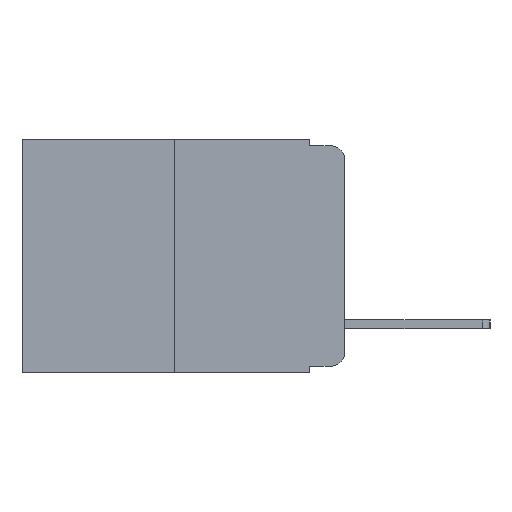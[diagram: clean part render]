
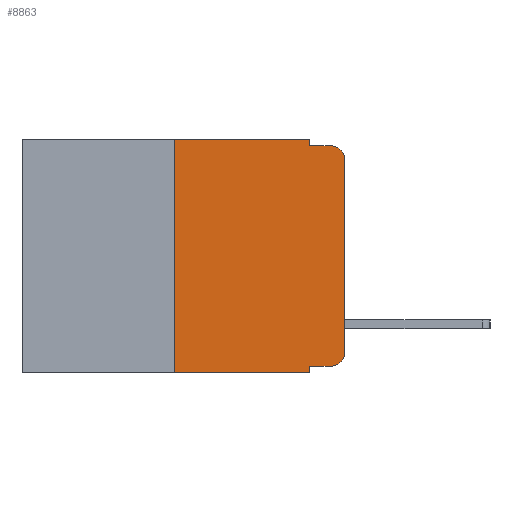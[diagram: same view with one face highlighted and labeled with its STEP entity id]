
A CAD part, left-side view. The second image highlights one B-rep face of the part: STEP entity #8863.
In plain terms, the highlighted planar face has unit normal (-1, 0, 0).
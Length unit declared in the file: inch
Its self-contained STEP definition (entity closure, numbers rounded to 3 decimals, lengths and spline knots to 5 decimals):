
#88 = EDGE_CURVE ( 'NONE', #5601, #2512, #3696, .T. ) ;
#154 = CARTESIAN_POINT ( 'NONE',  ( 0., 0., -0.313 ) ) ;
#872 = CARTESIAN_POINT ( 'NONE',  ( 0., 0.051, -0.343 ) ) ;
#1661 = EDGE_CURVE ( 'NONE', #13892, #5601, #1876, .T. ) ;
#1876 = LINE ( 'NONE', #6268, #14710 ) ;
#1945 = DIRECTION ( 'NONE',  ( 1., 0., 0. ) ) ;
#2285 = VERTEX_POINT ( 'NONE', #15141 ) ;
#2512 = VERTEX_POINT ( 'NONE', #3735 ) ;
#2529 = VECTOR ( 'NONE', #13108, 39.37008 ) ;
#2612 = AXIS2_PLACEMENT_3D ( 'NONE', #18096, #9336, #19507 ) ;
#2940 = CARTESIAN_POINT ( 'NONE',  ( 0., 0.051, 0. ) ) ;
#3211 = VECTOR ( 'NONE', #10409, 39.37008 ) ;
#3261 = AXIS2_PLACEMENT_3D ( 'NONE', #14001, #4772, #15434 ) ;
#3561 = ORIENTED_EDGE ( 'NONE', *, *, #1661, .F. ) ;
#3588 = CARTESIAN_POINT ( 'NONE',  ( 0., 0.473, -0.343 ) ) ;
#3696 = LINE ( 'NONE', #9716, #3211 ) ;
#3728 = CARTESIAN_POINT ( 'NONE',  ( 0., 0.051, 0. ) ) ;
#3735 = CARTESIAN_POINT ( 'NONE',  ( 0., 0.051, -0.01 ) ) ;
#3937 = CARTESIAN_POINT ( 'NONE',  ( 0., 0.02, -0.01 ) ) ;
#4514 = VERTEX_POINT ( 'NONE', #154 ) ;
#4584 = DIRECTION ( 'NONE',  ( 0., 0., 1. ) ) ;
#4772 = DIRECTION ( 'NONE',  ( -1., 0., 0. ) ) ;
#5089 = EDGE_CURVE ( 'NONE', #13348, #15191, #10966, .T. ) ;
#5204 = VERTEX_POINT ( 'NONE', #11725 ) ;
#5223 = VERTEX_POINT ( 'NONE', #3937 ) ;
#5286 = AXIS2_PLACEMENT_3D ( 'NONE', #11363, #1945, #12857 ) ;
#5326 = DIRECTION ( 'NONE',  ( 0., 0., -1. ) ) ;
#5601 = VERTEX_POINT ( 'NONE', #2940 ) ;
#5834 = VERTEX_POINT ( 'NONE', #8390 ) ;
#6155 = EDGE_CURVE ( 'NONE', #4514, #5834, #17070, .T. ) ;
#6268 = CARTESIAN_POINT ( 'NONE',  ( 0., 0.473, 0. ) ) ;
#6308 = ORIENTED_EDGE ( 'NONE', *, *, #14175, .F. ) ;
#6772 = LINE ( 'NONE', #17369, #2529 ) ;
#6827 = VECTOR ( 'NONE', #18651, 39.37008 ) ;
#7703 = CARTESIAN_POINT ( 'NONE',  ( 0., 0., 0. ) ) ;
#7787 = ORIENTED_EDGE ( 'NONE', *, *, #7931, .F. ) ;
#7931 = EDGE_CURVE ( 'NONE', #13348, #13892, #17855, .T. ) ;
#7959 = EDGE_CURVE ( 'NONE', #5204, #2285, #17402, .T. ) ;
#8142 = EDGE_CURVE ( 'NONE', #5834, #5223, #8359, .T. ) ;
#8277 = ORIENTED_EDGE ( 'NONE', *, *, #5089, .T. ) ;
#8359 = CIRCLE ( 'NONE', #2612, 0.02 ) ;
#8390 = CARTESIAN_POINT ( 'NONE',  ( 0., 0., -0.03 ) ) ;
#8511 = ORIENTED_EDGE ( 'NONE', *, *, #6155, .T. ) ;
#8863 = ADVANCED_FACE ( 'NONE', ( #13213 ), #15722, .F. ) ;
#9114 = VECTOR ( 'NONE', #18960, 39.37008 ) ;
#9336 = DIRECTION ( 'NONE',  ( -1., 0., 0. ) ) ;
#9351 = LINE ( 'NONE', #3728, #17171 ) ;
#9716 = CARTESIAN_POINT ( 'NONE',  ( 0., 0.051, 0. ) ) ;
#9719 = VECTOR ( 'NONE', #4584, 39.37008 ) ;
#10229 = ORIENTED_EDGE ( 'NONE', *, *, #14924, .T. ) ;
#10314 = DIRECTION ( 'NONE',  ( 0., -1., 0. ) ) ;
#10409 = DIRECTION ( 'NONE',  ( 0., 0., -1. ) ) ;
#10772 = EDGE_CURVE ( 'NONE', #5204, #15191, #9351, .T. ) ;
#10966 = LINE ( 'NONE', #3588, #6827 ) ;
#11363 = CARTESIAN_POINT ( 'NONE',  ( 0., 0.473, 0. ) ) ;
#11725 = CARTESIAN_POINT ( 'NONE',  ( 0., 0.051, -0.333 ) ) ;
#12811 = ORIENTED_EDGE ( 'NONE', *, *, #10772, .F. ) ;
#12857 = DIRECTION ( 'NONE',  ( 0., 0., -1. ) ) ;
#13108 = DIRECTION ( 'NONE',  ( 0., -1., 0. ) ) ;
#13171 = CARTESIAN_POINT ( 'NONE',  ( 0., 0.25, 0. ) ) ;
#13213 = FACE_OUTER_BOUND ( 'NONE', #15554, .T. ) ;
#13348 = VERTEX_POINT ( 'NONE', #13803 ) ;
#13569 = CIRCLE ( 'NONE', #3261, 0.02 ) ;
#13616 = VECTOR ( 'NONE', #14641, 39.37008 ) ;
#13803 = CARTESIAN_POINT ( 'NONE',  ( 0., 0.25, -0.343 ) ) ;
#13846 = CARTESIAN_POINT ( 'NONE',  ( 0., 0.25, 0. ) ) ;
#13892 = VERTEX_POINT ( 'NONE', #13846 ) ;
#14001 = CARTESIAN_POINT ( 'NONE',  ( 0., 0.02, -0.313 ) ) ;
#14175 = EDGE_CURVE ( 'NONE', #2512, #5223, #6772, .T. ) ;
#14641 = DIRECTION ( 'NONE',  ( 0., 0., 1. ) ) ;
#14701 = CARTESIAN_POINT ( 'NONE',  ( 0., 0.051, -0.333 ) ) ;
#14710 = VECTOR ( 'NONE', #10314, 39.37008 ) ;
#14924 = EDGE_CURVE ( 'NONE', #2285, #4514, #13569, .T. ) ;
#15141 = CARTESIAN_POINT ( 'NONE',  ( 0., 0.02, -0.333 ) ) ;
#15191 = VERTEX_POINT ( 'NONE', #872 ) ;
#15434 = DIRECTION ( 'NONE',  ( 0., 0., -1. ) ) ;
#15554 = EDGE_LOOP ( 'NONE', ( #8511, #16427, #6308, #19067, #3561, #7787, #8277, #12811, #17103, #10229 ) ) ;
#15722 = PLANE ( 'NONE',  #5286 ) ;
#16427 = ORIENTED_EDGE ( 'NONE', *, *, #8142, .T. ) ;
#17070 = LINE ( 'NONE', #7703, #9719 ) ;
#17103 = ORIENTED_EDGE ( 'NONE', *, *, #7959, .T. ) ;
#17171 = VECTOR ( 'NONE', #5326, 39.37008 ) ;
#17369 = CARTESIAN_POINT ( 'NONE',  ( 0., 0.051, -0.01 ) ) ;
#17402 = LINE ( 'NONE', #14701, #9114 ) ;
#17855 = LINE ( 'NONE', #13171, #13616 ) ;
#18096 = CARTESIAN_POINT ( 'NONE',  ( 0., 0.02, -0.03 ) ) ;
#18651 = DIRECTION ( 'NONE',  ( 0., -1., 0. ) ) ;
#18960 = DIRECTION ( 'NONE',  ( 0., -1., 0. ) ) ;
#19067 = ORIENTED_EDGE ( 'NONE', *, *, #88, .F. ) ;
#19507 = DIRECTION ( 'NONE',  ( 0., 0., -1. ) ) ;
